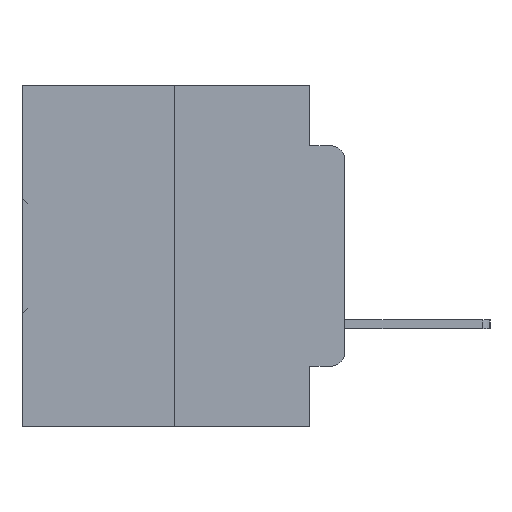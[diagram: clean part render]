
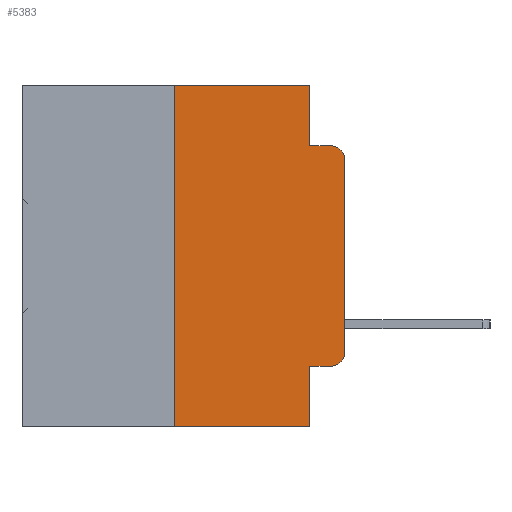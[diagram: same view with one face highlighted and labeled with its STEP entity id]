
A CAD part, left-side view. The second image highlights one B-rep face of the part: STEP entity #5383.
In plain terms, the highlighted planar face has unit normal (-1, 0, 0).
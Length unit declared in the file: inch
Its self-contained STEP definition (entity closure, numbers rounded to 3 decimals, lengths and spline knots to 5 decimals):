
#66 = LINE ( 'NONE', #14688, #27723 ) ;
#705 = CARTESIAN_POINT ( 'NONE',  ( 0., 0.25, 0. ) ) ;
#1466 = ORIENTED_EDGE ( 'NONE', *, *, #14256, .F. ) ;
#1526 = FACE_OUTER_BOUND ( 'NONE', #5895, .T. ) ;
#1610 = DIRECTION ( 'NONE',  ( 0., -1., 0. ) ) ;
#1611 = ORIENTED_EDGE ( 'NONE', *, *, #11864, .T. ) ;
#1983 = VERTEX_POINT ( 'NONE', #34457 ) ;
#2471 = VECTOR ( 'NONE', #18580, 39.37008 ) ;
#3249 = CARTESIAN_POINT ( 'NONE',  ( 0., 0.473, 0. ) ) ;
#3333 = EDGE_CURVE ( 'NONE', #4021, #30218, #30495, .T. ) ;
#3395 = CARTESIAN_POINT ( 'NONE',  ( 0., 0.051, -0.0885 ) ) ;
#3397 = PLANE ( 'NONE',  #3661 ) ;
#3576 = ORIENTED_EDGE ( 'NONE', *, *, #12166, .F. ) ;
#3589 = DIRECTION ( 'NONE',  ( 0., 0., -1. ) ) ;
#3661 = AXIS2_PLACEMENT_3D ( 'NONE', #3249, #6888, #3589 ) ;
#3998 = LINE ( 'NONE', #705, #25406 ) ;
#4021 = VERTEX_POINT ( 'NONE', #27568 ) ;
#4156 = LINE ( 'NONE', #26380, #31695 ) ;
#4392 = VECTOR ( 'NONE', #25679, 39.37008 ) ;
#5190 = CARTESIAN_POINT ( 'NONE',  ( 0., 0.25, 0. ) ) ;
#5383 = ADVANCED_FACE ( 'NONE', ( #1526 ), #3397, .F. ) ;
#5639 = ORIENTED_EDGE ( 'NONE', *, *, #12365, .T. ) ;
#5749 = ORIENTED_EDGE ( 'NONE', *, *, #9232, .T. ) ;
#5872 = VECTOR ( 'NONE', #1610, 39.37008 ) ;
#5895 = EDGE_LOOP ( 'NONE', ( #22387, #23113, #20377, #27829, #1466, #3576, #5749, #24032, #5639, #1611 ) ) ;
#6266 = VERTEX_POINT ( 'NONE', #11533 ) ;
#6888 = DIRECTION ( 'NONE',  ( 1., 0., 0. ) ) ;
#6911 = CARTESIAN_POINT ( 'NONE',  ( 0., 0.051, -0.4115 ) ) ;
#7805 = CIRCLE ( 'NONE', #34323, 0.02 ) ;
#8101 = VERTEX_POINT ( 'NONE', #5190 ) ;
#9189 = EDGE_CURVE ( 'NONE', #32730, #29811, #4156, .T. ) ;
#9232 = EDGE_CURVE ( 'NONE', #20447, #29811, #23920, .T. ) ;
#10280 = DIRECTION ( 'NONE',  ( -1., 0., 0. ) ) ;
#10322 = LINE ( 'NONE', #21489, #24557 ) ;
#10836 = DIRECTION ( 'NONE',  ( 0., 0., 1. ) ) ;
#11533 = CARTESIAN_POINT ( 'NONE',  ( 0., 0.02, -0.4115 ) ) ;
#11864 = EDGE_CURVE ( 'NONE', #6266, #1983, #7805, .T. ) ;
#12040 = CARTESIAN_POINT ( 'NONE',  ( 0., 0.051, -0.4115 ) ) ;
#12166 = EDGE_CURVE ( 'NONE', #20447, #8101, #3998, .T. ) ;
#12184 = VERTEX_POINT ( 'NONE', #3395 ) ;
#12365 = EDGE_CURVE ( 'NONE', #32730, #6266, #25816, .T. ) ;
#12626 = EDGE_CURVE ( 'NONE', #32091, #12184, #10322, .T. ) ;
#13094 = LINE ( 'NONE', #33523, #5872 ) ;
#14256 = EDGE_CURVE ( 'NONE', #8101, #32091, #66, .T. ) ;
#14688 = CARTESIAN_POINT ( 'NONE',  ( 0., 0.473, 0. ) ) ;
#15566 = CARTESIAN_POINT ( 'NONE',  ( 0., 0.02, -0.3915 ) ) ;
#15690 = VECTOR ( 'NONE', #10836, 39.37008 ) ;
#15899 = CARTESIAN_POINT ( 'NONE',  ( 0., 0.473, -0.5 ) ) ;
#16207 = CARTESIAN_POINT ( 'NONE',  ( 0., 0., 0. ) ) ;
#16705 = CARTESIAN_POINT ( 'NONE',  ( 0., 0.02, -0.0885 ) ) ;
#17684 = CARTESIAN_POINT ( 'NONE',  ( 0., 0.051, -0.5 ) ) ;
#18241 = DIRECTION ( 'NONE',  ( 0., 0., -1. ) ) ;
#18580 = DIRECTION ( 'NONE',  ( 0., -1., 0. ) ) ;
#18844 = CARTESIAN_POINT ( 'NONE',  ( 0., 0.25, -0.5 ) ) ;
#19518 = DIRECTION ( 'NONE',  ( 0., 0., 1. ) ) ;
#20377 = ORIENTED_EDGE ( 'NONE', *, *, #33892, .F. ) ;
#20447 = VERTEX_POINT ( 'NONE', #18844 ) ;
#21489 = CARTESIAN_POINT ( 'NONE',  ( 0., 0.051, 0. ) ) ;
#22387 = ORIENTED_EDGE ( 'NONE', *, *, #33060, .T. ) ;
#22636 = CARTESIAN_POINT ( 'NONE',  ( 0., 0.051, 0. ) ) ;
#23113 = ORIENTED_EDGE ( 'NONE', *, *, #3333, .T. ) ;
#23920 = LINE ( 'NONE', #15899, #2471 ) ;
#24032 = ORIENTED_EDGE ( 'NONE', *, *, #9189, .F. ) ;
#24557 = VECTOR ( 'NONE', #31930, 39.37008 ) ;
#25293 = DIRECTION ( 'NONE',  ( 0., -1., 0. ) ) ;
#25406 = VECTOR ( 'NONE', #19518, 39.37008 ) ;
#25679 = DIRECTION ( 'NONE',  ( 0., -1., 0. ) ) ;
#25816 = LINE ( 'NONE', #6911, #4392 ) ;
#26380 = CARTESIAN_POINT ( 'NONE',  ( 0., 0.051, 0. ) ) ;
#27568 = CARTESIAN_POINT ( 'NONE',  ( 0., 0., -0.1085 ) ) ;
#27723 = VECTOR ( 'NONE', #25293, 39.37008 ) ;
#27829 = ORIENTED_EDGE ( 'NONE', *, *, #12626, .F. ) ;
#29013 = DIRECTION ( 'NONE',  ( 0., 0., -1. ) ) ;
#29772 = LINE ( 'NONE', #16207, #15690 ) ;
#29811 = VERTEX_POINT ( 'NONE', #17684 ) ;
#29967 = AXIS2_PLACEMENT_3D ( 'NONE', #33558, #10280, #32240 ) ;
#30218 = VERTEX_POINT ( 'NONE', #16705 ) ;
#30495 = CIRCLE ( 'NONE', #29967, 0.02 ) ;
#31695 = VECTOR ( 'NONE', #29013, 39.37008 ) ;
#31930 = DIRECTION ( 'NONE',  ( 0., 0., -1. ) ) ;
#32091 = VERTEX_POINT ( 'NONE', #22636 ) ;
#32240 = DIRECTION ( 'NONE',  ( 0., 0., -1. ) ) ;
#32730 = VERTEX_POINT ( 'NONE', #12040 ) ;
#33060 = EDGE_CURVE ( 'NONE', #1983, #4021, #29772, .T. ) ;
#33523 = CARTESIAN_POINT ( 'NONE',  ( 0., 0.051, -0.0885 ) ) ;
#33558 = CARTESIAN_POINT ( 'NONE',  ( 0., 0.02, -0.1085 ) ) ;
#33892 = EDGE_CURVE ( 'NONE', #12184, #30218, #13094, .T. ) ;
#34041 = DIRECTION ( 'NONE',  ( -1., 0., 0. ) ) ;
#34323 = AXIS2_PLACEMENT_3D ( 'NONE', #15566, #34041, #18241 ) ;
#34457 = CARTESIAN_POINT ( 'NONE',  ( 0., 0., -0.3915 ) ) ;
